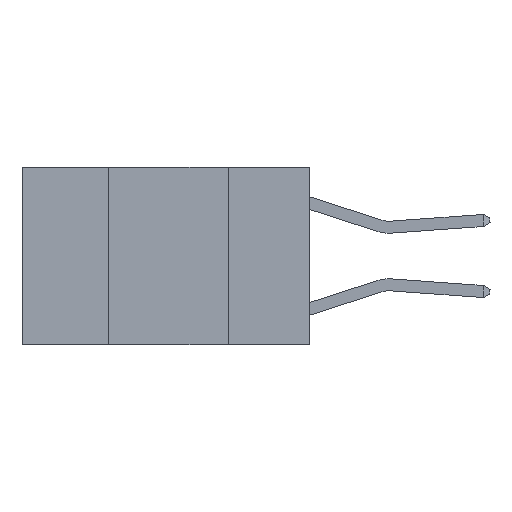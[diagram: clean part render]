
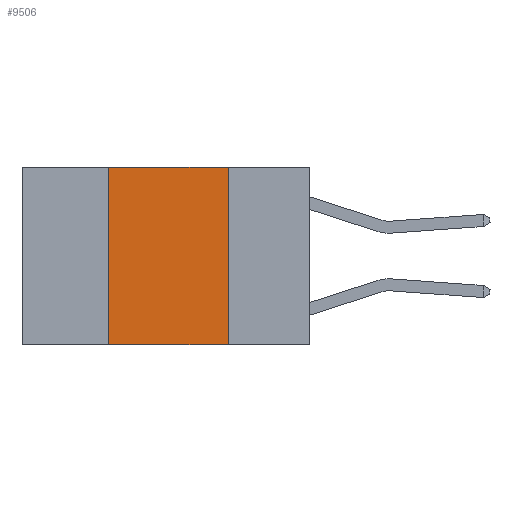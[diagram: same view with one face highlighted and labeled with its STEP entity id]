
A CAD part, left-side view. The second image highlights one B-rep face of the part: STEP entity #9506.
In plain terms, the highlighted planar face has unit normal (-1, 0, 0).
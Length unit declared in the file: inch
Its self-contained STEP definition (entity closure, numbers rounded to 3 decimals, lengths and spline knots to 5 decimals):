
#131 = CARTESIAN_POINT ( 'NONE',  ( 0., 0.6, 0. ) ) ;
#407 = DIRECTION ( 'NONE',  ( 1., 0., 0. ) ) ;
#511 = CARTESIAN_POINT ( 'NONE',  ( 0., 0.17, 0. ) ) ;
#1188 = DIRECTION ( 'NONE',  ( 0., -1., 0. ) ) ;
#1252 = EDGE_CURVE ( 'NONE', #14807, #16990, #3872, .T. ) ;
#1458 = LINE ( 'NONE', #131, #1505 ) ;
#1505 = VECTOR ( 'NONE', #1188, 39.37008 ) ;
#2639 = CARTESIAN_POINT ( 'NONE',  ( 0., 0.17, 0. ) ) ;
#2989 = EDGE_CURVE ( 'NONE', #14807, #9097, #6465, .T. ) ;
#3554 = EDGE_CURVE ( 'NONE', #5099, #9097, #6704, .T. ) ;
#3872 = LINE ( 'NONE', #10687, #4977 ) ;
#3902 = CARTESIAN_POINT ( 'NONE',  ( 0., 0.42, 0. ) ) ;
#3962 = ORIENTED_EDGE ( 'NONE', *, *, #1252, .F. ) ;
#4547 = DIRECTION ( 'NONE',  ( 0., 0., -1. ) ) ;
#4977 = VECTOR ( 'NONE', #7858, 39.37008 ) ;
#5099 = VERTEX_POINT ( 'NONE', #511 ) ;
#5128 = CARTESIAN_POINT ( 'NONE',  ( 0., 0.6, -0.37 ) ) ;
#5404 = VECTOR ( 'NONE', #13357, 39.37008 ) ;
#6465 = LINE ( 'NONE', #5128, #5404 ) ;
#6704 = LINE ( 'NONE', #2639, #16835 ) ;
#7858 = DIRECTION ( 'NONE',  ( 0., 0., 1. ) ) ;
#8464 = CARTESIAN_POINT ( 'NONE',  ( 0., 0.6, 0. ) ) ;
#8549 = CARTESIAN_POINT ( 'NONE',  ( 0., 0.42, -0.37 ) ) ;
#9097 = VERTEX_POINT ( 'NONE', #9659 ) ;
#9506 = ADVANCED_FACE ( 'NONE', ( #12340 ), #10934, .F. ) ;
#9659 = CARTESIAN_POINT ( 'NONE',  ( 0., 0.17, -0.37 ) ) ;
#10687 = CARTESIAN_POINT ( 'NONE',  ( 0., 0.42, 0. ) ) ;
#10822 = ORIENTED_EDGE ( 'NONE', *, *, #14752, .F. ) ;
#10934 = PLANE ( 'NONE',  #17206 ) ;
#11991 = ORIENTED_EDGE ( 'NONE', *, *, #2989, .T. ) ;
#12340 = FACE_OUTER_BOUND ( 'NONE', #15996, .T. ) ;
#12451 = DIRECTION ( 'NONE',  ( 0., 0., -1. ) ) ;
#13357 = DIRECTION ( 'NONE',  ( 0., -1., 0. ) ) ;
#14708 = ORIENTED_EDGE ( 'NONE', *, *, #3554, .F. ) ;
#14752 = EDGE_CURVE ( 'NONE', #16990, #5099, #1458, .T. ) ;
#14807 = VERTEX_POINT ( 'NONE', #8549 ) ;
#15996 = EDGE_LOOP ( 'NONE', ( #14708, #10822, #3962, #11991 ) ) ;
#16835 = VECTOR ( 'NONE', #12451, 39.37008 ) ;
#16990 = VERTEX_POINT ( 'NONE', #3902 ) ;
#17206 = AXIS2_PLACEMENT_3D ( 'NONE', #8464, #407, #4547 ) ;
